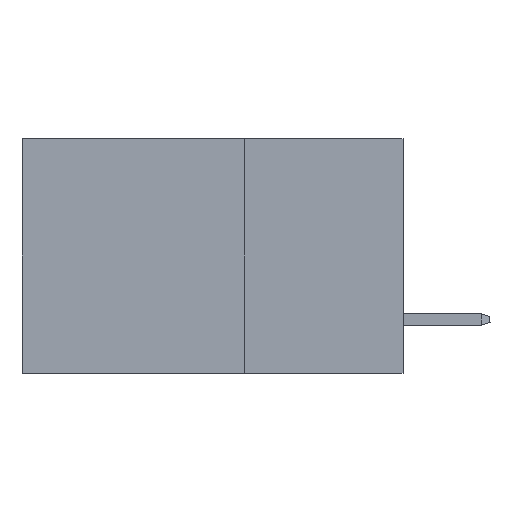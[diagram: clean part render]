
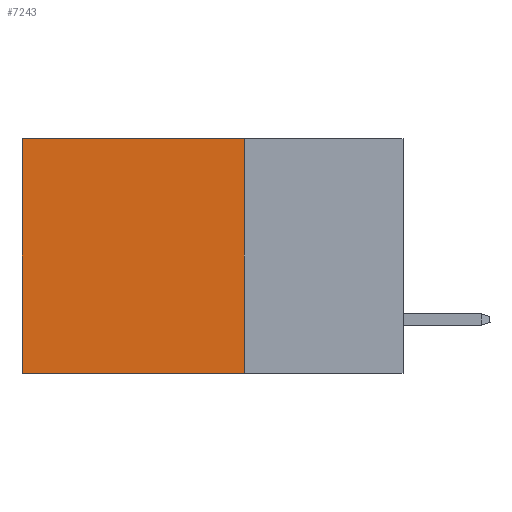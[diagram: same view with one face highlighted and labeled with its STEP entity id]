
A CAD part, left-side view. The second image highlights one B-rep face of the part: STEP entity #7243.
In plain terms, the highlighted planar face has unit normal (-1, 0, 0).
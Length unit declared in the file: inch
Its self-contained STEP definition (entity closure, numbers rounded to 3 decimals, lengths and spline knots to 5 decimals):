
#47 = PLANE ( 'NONE',  #17178 ) ;
#492 = ORIENTED_EDGE ( 'NONE', *, *, #11963, .T. ) ;
#744 = EDGE_CURVE ( 'NONE', #11028, #5834, #15182, .T. ) ;
#832 = LINE ( 'NONE', #11672, #4470 ) ;
#1290 = VECTOR ( 'NONE', #14363, 39.37008 ) ;
#2068 = LINE ( 'NONE', #7836, #1290 ) ;
#2869 = ORIENTED_EDGE ( 'NONE', *, *, #15821, .F. ) ;
#3538 = ORIENTED_EDGE ( 'NONE', *, *, #744, .T. ) ;
#4470 = VECTOR ( 'NONE', #16270, 39.37008 ) ;
#5834 = VERTEX_POINT ( 'NONE', #17789 ) ;
#6185 = CARTESIAN_POINT ( 'NONE',  ( 0.2875, 0.25, 0. ) ) ;
#6389 = FACE_OUTER_BOUND ( 'NONE', #8158, .T. ) ;
#7243 = ADVANCED_FACE ( 'NONE', ( #6389 ), #47, .F. ) ;
#7586 = CARTESIAN_POINT ( 'NONE',  ( 0.2875, 0.6, -0.37 ) ) ;
#7640 = VECTOR ( 'NONE', #9693, 39.37008 ) ;
#7836 = CARTESIAN_POINT ( 'NONE',  ( 0.2875, 0.25, -0.37 ) ) ;
#8158 = EDGE_LOOP ( 'NONE', ( #492, #19194, #2869, #3538 ) ) ;
#9693 = DIRECTION ( 'NONE',  ( 0., 0., -1. ) ) ;
#10333 = CARTESIAN_POINT ( 'NONE',  ( 0.2875, 0.25, 0. ) ) ;
#10686 = CARTESIAN_POINT ( 'NONE',  ( 0.2875, 0.25, 0. ) ) ;
#11028 = VERTEX_POINT ( 'NONE', #10333 ) ;
#11672 = CARTESIAN_POINT ( 'NONE',  ( 0.2875, 0.25, 0. ) ) ;
#11963 = EDGE_CURVE ( 'NONE', #5834, #18787, #17302, .T. ) ;
#12096 = DIRECTION ( 'NONE',  ( 0., 1., 0. ) ) ;
#13301 = CARTESIAN_POINT ( 'NONE',  ( 0.2875, 0.25, -0.37 ) ) ;
#14363 = DIRECTION ( 'NONE',  ( 0., 1., 0. ) ) ;
#15182 = LINE ( 'NONE', #10686, #16364 ) ;
#15673 = DIRECTION ( 'NONE',  ( 1., 0., 0. ) ) ;
#15821 = EDGE_CURVE ( 'NONE', #11028, #19139, #832, .T. ) ;
#16270 = DIRECTION ( 'NONE',  ( 0., 0., -1. ) ) ;
#16364 = VECTOR ( 'NONE', #12096, 39.37008 ) ;
#17178 = AXIS2_PLACEMENT_3D ( 'NONE', #6185, #15673, #17188 ) ;
#17188 = DIRECTION ( 'NONE',  ( 0., 0., -1. ) ) ;
#17302 = LINE ( 'NONE', #17399, #7640 ) ;
#17399 = CARTESIAN_POINT ( 'NONE',  ( 0.2875, 0.6, 0. ) ) ;
#17789 = CARTESIAN_POINT ( 'NONE',  ( 0.2875, 0.6, 0. ) ) ;
#18787 = VERTEX_POINT ( 'NONE', #7586 ) ;
#19139 = VERTEX_POINT ( 'NONE', #13301 ) ;
#19194 = ORIENTED_EDGE ( 'NONE', *, *, #19498, .F. ) ;
#19498 = EDGE_CURVE ( 'NONE', #19139, #18787, #2068, .T. ) ;
